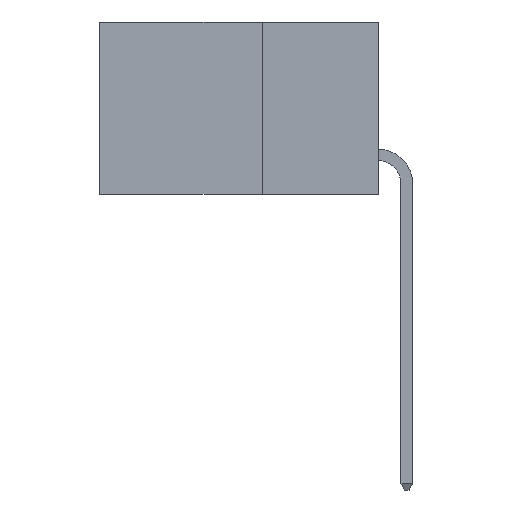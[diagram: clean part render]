
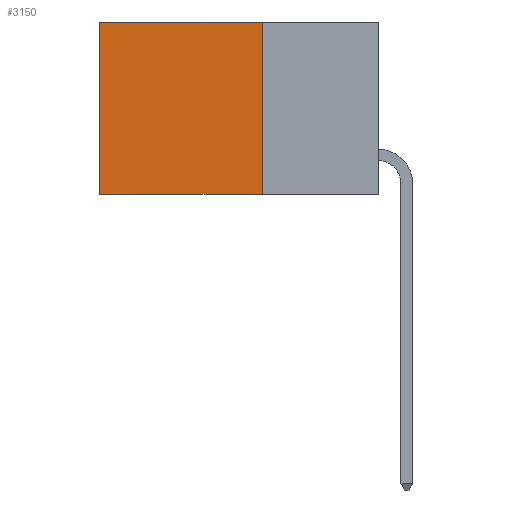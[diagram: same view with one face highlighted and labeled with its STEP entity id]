
A CAD part, left-side view. The second image highlights one B-rep face of the part: STEP entity #3150.
In plain terms, the highlighted planar face has unit normal (-1, 0, 0).
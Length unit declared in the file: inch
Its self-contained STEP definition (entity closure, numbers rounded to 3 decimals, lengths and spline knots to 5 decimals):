
#465 = LINE ( 'NONE', #9055, #5031 ) ;
#633 = DIRECTION ( 'NONE',  ( 0., 0., -1. ) ) ;
#713 = CARTESIAN_POINT ( 'NONE',  ( 0.2615, 0.25, -0.37 ) ) ;
#958 = VECTOR ( 'NONE', #19392, 39.37008 ) ;
#1853 = EDGE_CURVE ( 'NONE', #10449, #15212, #5862, .T. ) ;
#2538 = CARTESIAN_POINT ( 'NONE',  ( 0.2615, 0.6, -0.37 ) ) ;
#3126 = VERTEX_POINT ( 'NONE', #11416 ) ;
#3150 = ADVANCED_FACE ( 'NONE', ( #5171 ), #10995, .F. ) ;
#3294 = DIRECTION ( 'NONE',  ( 0., 1., 0. ) ) ;
#3404 = CARTESIAN_POINT ( 'NONE',  ( 0.2615, 0.25, 0. ) ) ;
#5031 = VECTOR ( 'NONE', #3294, 39.37008 ) ;
#5171 = FACE_OUTER_BOUND ( 'NONE', #16674, .T. ) ;
#5242 = VECTOR ( 'NONE', #633, 39.37008 ) ;
#5862 = LINE ( 'NONE', #713, #5242 ) ;
#8022 = CARTESIAN_POINT ( 'NONE',  ( 0.2615, 0.25, -0.37 ) ) ;
#8050 = VECTOR ( 'NONE', #20382, 39.37008 ) ;
#8488 = ORIENTED_EDGE ( 'NONE', *, *, #11041, .F. ) ;
#9055 = CARTESIAN_POINT ( 'NONE',  ( 0.2615, 0.25, -0.37 ) ) ;
#10449 = VERTEX_POINT ( 'NONE', #3404 ) ;
#10482 = ORIENTED_EDGE ( 'NONE', *, *, #1853, .F. ) ;
#10884 = DIRECTION ( 'NONE',  ( 0., 0., -1. ) ) ;
#10915 = DIRECTION ( 'NONE',  ( 1., 0., 0. ) ) ;
#10967 = CARTESIAN_POINT ( 'NONE',  ( 0.2615, 0.25, -0.37 ) ) ;
#10995 = PLANE ( 'NONE',  #19336 ) ;
#11041 = EDGE_CURVE ( 'NONE', #15212, #19032, #465, .T. ) ;
#11416 = CARTESIAN_POINT ( 'NONE',  ( 0.2615, 0.6, 0. ) ) ;
#11780 = EDGE_CURVE ( 'NONE', #3126, #19032, #23436, .T. ) ;
#13497 = ORIENTED_EDGE ( 'NONE', *, *, #20232, .T. ) ;
#15212 = VERTEX_POINT ( 'NONE', #8022 ) ;
#16674 = EDGE_LOOP ( 'NONE', ( #17494, #8488, #10482, #13497 ) ) ;
#17491 = CARTESIAN_POINT ( 'NONE',  ( 0.2615, 0.25, 0. ) ) ;
#17494 = ORIENTED_EDGE ( 'NONE', *, *, #11780, .T. ) ;
#19032 = VERTEX_POINT ( 'NONE', #2538 ) ;
#19336 = AXIS2_PLACEMENT_3D ( 'NONE', #10967, #10915, #10884 ) ;
#19392 = DIRECTION ( 'NONE',  ( 0., 1., 0. ) ) ;
#20232 = EDGE_CURVE ( 'NONE', #10449, #3126, #20365, .T. ) ;
#20365 = LINE ( 'NONE', #17491, #958 ) ;
#20382 = DIRECTION ( 'NONE',  ( 0., 0., -1. ) ) ;
#23436 = LINE ( 'NONE', #24216, #8050 ) ;
#24216 = CARTESIAN_POINT ( 'NONE',  ( 0.2615, 0.6, -0.37 ) ) ;
